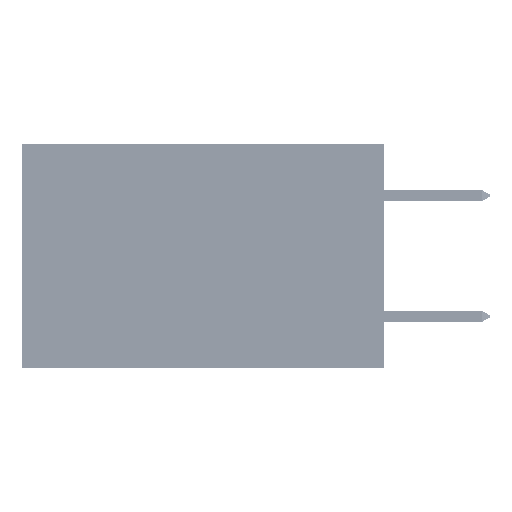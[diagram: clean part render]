
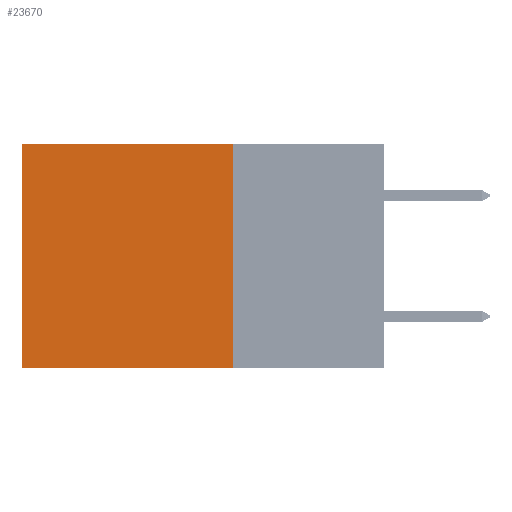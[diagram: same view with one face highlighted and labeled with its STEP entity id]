
A CAD part, left-side view. The second image highlights one B-rep face of the part: STEP entity #23670.
In plain terms, the highlighted planar face has unit normal (-1, 0, 0).
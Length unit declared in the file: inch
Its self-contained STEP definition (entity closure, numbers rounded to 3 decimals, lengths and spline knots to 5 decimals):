
#332 = AXIS2_PLACEMENT_3D ( 'NONE', #7649, #51458, #19212 ) ;
#820 = DIRECTION ( 'NONE',  ( 0., 0., -1. ) ) ;
#5641 = EDGE_LOOP ( 'NONE', ( #14391, #6526, #30499, #13182 ) ) ;
#5787 = CARTESIAN_POINT ( 'NONE',  ( 0.2875, 0.25, -0.37 ) ) ;
#6526 = ORIENTED_EDGE ( 'NONE', *, *, #25950, .F. ) ;
#6776 = LINE ( 'NONE', #5787, #45071 ) ;
#7649 = CARTESIAN_POINT ( 'NONE',  ( 0.2875, 0.25, 0. ) ) ;
#13182 = ORIENTED_EDGE ( 'NONE', *, *, #15735, .T. ) ;
#14007 = LINE ( 'NONE', #27764, #51626 ) ;
#14343 = EDGE_CURVE ( 'NONE', #38443, #40467, #31069, .T. ) ;
#14391 = ORIENTED_EDGE ( 'NONE', *, *, #48612, .T. ) ;
#15529 = DIRECTION ( 'NONE',  ( 0., 1., 0. ) ) ;
#15735 = EDGE_CURVE ( 'NONE', #38443, #46639, #14007, .T. ) ;
#17149 = VECTOR ( 'NONE', #820, 39.37008 ) ;
#19212 = DIRECTION ( 'NONE',  ( 0., 0., -1. ) ) ;
#23670 = ADVANCED_FACE ( 'NONE', ( #33895 ), #43559, .F. ) ;
#25403 = CARTESIAN_POINT ( 'NONE',  ( 0.2875, 0.6, 0. ) ) ;
#25950 = EDGE_CURVE ( 'NONE', #40467, #26732, #6776, .T. ) ;
#26732 = VERTEX_POINT ( 'NONE', #50765 ) ;
#27764 = CARTESIAN_POINT ( 'NONE',  ( 0.2875, 0.25, 0. ) ) ;
#30398 = CARTESIAN_POINT ( 'NONE',  ( 0.2875, 0.25, 0. ) ) ;
#30499 = ORIENTED_EDGE ( 'NONE', *, *, #14343, .F. ) ;
#31069 = LINE ( 'NONE', #30398, #41070 ) ;
#33409 = LINE ( 'NONE', #25403, #17149 ) ;
#33895 = FACE_OUTER_BOUND ( 'NONE', #5641, .T. ) ;
#36618 = CARTESIAN_POINT ( 'NONE',  ( 0.2875, 0.25, 0. ) ) ;
#37596 = DIRECTION ( 'NONE',  ( 0., 0., -1. ) ) ;
#38443 = VERTEX_POINT ( 'NONE', #36618 ) ;
#40467 = VERTEX_POINT ( 'NONE', #45763 ) ;
#41070 = VECTOR ( 'NONE', #37596, 39.37008 ) ;
#43559 = PLANE ( 'NONE',  #332 ) ;
#45071 = VECTOR ( 'NONE', #46473, 39.37008 ) ;
#45763 = CARTESIAN_POINT ( 'NONE',  ( 0.2875, 0.25, -0.37 ) ) ;
#46473 = DIRECTION ( 'NONE',  ( 0., 1., 0. ) ) ;
#46639 = VERTEX_POINT ( 'NONE', #48186 ) ;
#48186 = CARTESIAN_POINT ( 'NONE',  ( 0.2875, 0.6, 0. ) ) ;
#48612 = EDGE_CURVE ( 'NONE', #46639, #26732, #33409, .T. ) ;
#50765 = CARTESIAN_POINT ( 'NONE',  ( 0.2875, 0.6, -0.37 ) ) ;
#51458 = DIRECTION ( 'NONE',  ( 1., 0., 0. ) ) ;
#51626 = VECTOR ( 'NONE', #15529, 39.37008 ) ;
